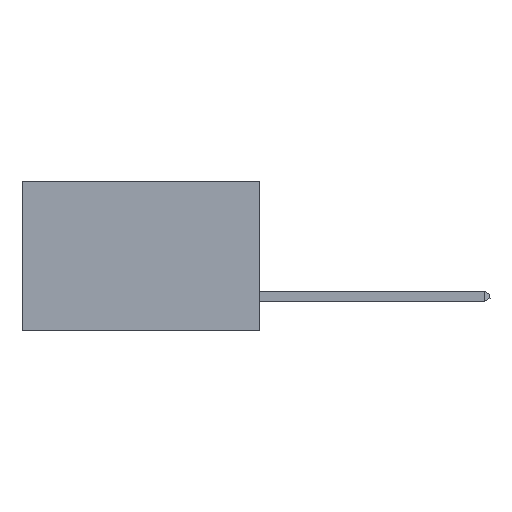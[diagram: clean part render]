
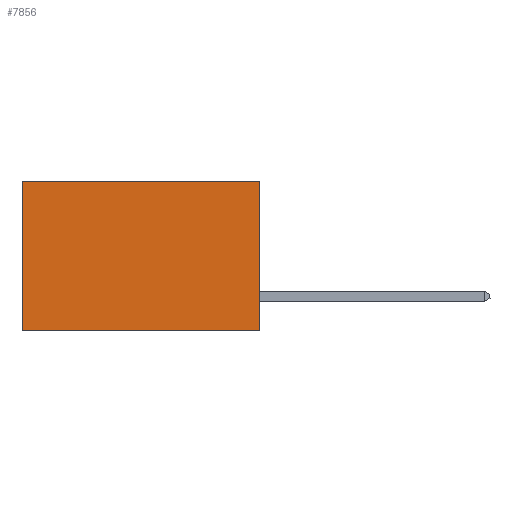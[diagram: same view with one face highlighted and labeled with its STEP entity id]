
A CAD part, left-side view. The second image highlights one B-rep face of the part: STEP entity #7856.
In plain terms, the highlighted planar face has unit normal (-1, 0, 0).
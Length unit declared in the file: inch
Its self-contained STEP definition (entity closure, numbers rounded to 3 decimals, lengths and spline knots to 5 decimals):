
#266 = CARTESIAN_POINT ( 'NONE',  ( 0.277, 0., -0.37 ) ) ;
#1131 = LINE ( 'NONE', #8456, #8256 ) ;
#1133 = DIRECTION ( 'NONE',  ( 0., 0., -1. ) ) ;
#1146 = DIRECTION ( 'NONE',  ( 1., 0., 0. ) ) ;
#1232 = CARTESIAN_POINT ( 'NONE',  ( 0.277, 0., -0.37 ) ) ;
#1267 = PLANE ( 'NONE',  #6358 ) ;
#1490 = EDGE_CURVE ( 'NONE', #7965, #4063, #1131, .T. ) ;
#2153 = CARTESIAN_POINT ( 'NONE',  ( 0.277, 0., 0. ) ) ;
#2754 = VERTEX_POINT ( 'NONE', #10633 ) ;
#2810 = LINE ( 'NONE', #3730, #4974 ) ;
#3373 = ORIENTED_EDGE ( 'NONE', *, *, #1490, .F. ) ;
#3453 = DIRECTION ( 'NONE',  ( 0., 0., -1. ) ) ;
#3730 = CARTESIAN_POINT ( 'NONE',  ( 0.277, 0.59, -0.37 ) ) ;
#4063 = VERTEX_POINT ( 'NONE', #5980 ) ;
#4134 = ORIENTED_EDGE ( 'NONE', *, *, #7575, .T. ) ;
#4827 = FACE_OUTER_BOUND ( 'NONE', #4975, .T. ) ;
#4847 = EDGE_CURVE ( 'NONE', #7728, #2754, #9254, .T. ) ;
#4974 = VECTOR ( 'NONE', #3453, 39.37008 ) ;
#4975 = EDGE_LOOP ( 'NONE', ( #4134, #3373, #5669, #7875 ) ) ;
#5291 = VECTOR ( 'NONE', #9641, 39.37008 ) ;
#5569 = LINE ( 'NONE', #9834, #5291 ) ;
#5627 = EDGE_CURVE ( 'NONE', #7728, #7965, #5569, .T. ) ;
#5669 = ORIENTED_EDGE ( 'NONE', *, *, #5627, .F. ) ;
#5980 = CARTESIAN_POINT ( 'NONE',  ( 0.277, 0.59, -0.37 ) ) ;
#6358 = AXIS2_PLACEMENT_3D ( 'NONE', #1232, #1146, #1133 ) ;
#6865 = VECTOR ( 'NONE', #9973, 39.37008 ) ;
#7575 = EDGE_CURVE ( 'NONE', #2754, #4063, #2810, .T. ) ;
#7728 = VERTEX_POINT ( 'NONE', #2153 ) ;
#7856 = ADVANCED_FACE ( 'NONE', ( #4827 ), #1267, .F. ) ;
#7875 = ORIENTED_EDGE ( 'NONE', *, *, #4847, .T. ) ;
#7965 = VERTEX_POINT ( 'NONE', #266 ) ;
#8045 = DIRECTION ( 'NONE',  ( 0., 1., 0. ) ) ;
#8256 = VECTOR ( 'NONE', #8045, 39.37008 ) ;
#8456 = CARTESIAN_POINT ( 'NONE',  ( 0.277, 0., -0.37 ) ) ;
#9254 = LINE ( 'NONE', #9958, #6865 ) ;
#9641 = DIRECTION ( 'NONE',  ( 0., 0., -1. ) ) ;
#9834 = CARTESIAN_POINT ( 'NONE',  ( 0.277, 0., -0.37 ) ) ;
#9958 = CARTESIAN_POINT ( 'NONE',  ( 0.277, 0., 0. ) ) ;
#9973 = DIRECTION ( 'NONE',  ( 0., 1., 0. ) ) ;
#10633 = CARTESIAN_POINT ( 'NONE',  ( 0.277, 0.59, 0. ) ) ;
